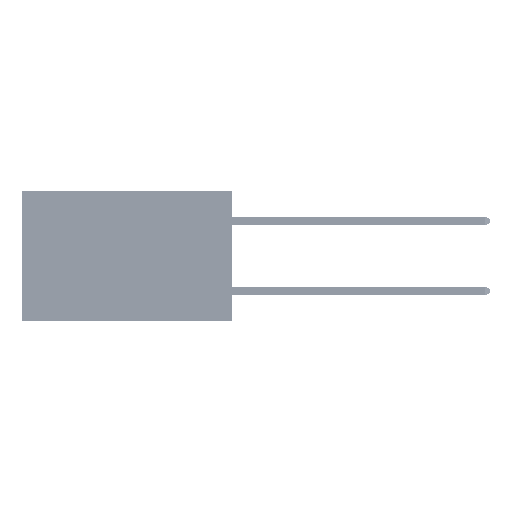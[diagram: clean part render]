
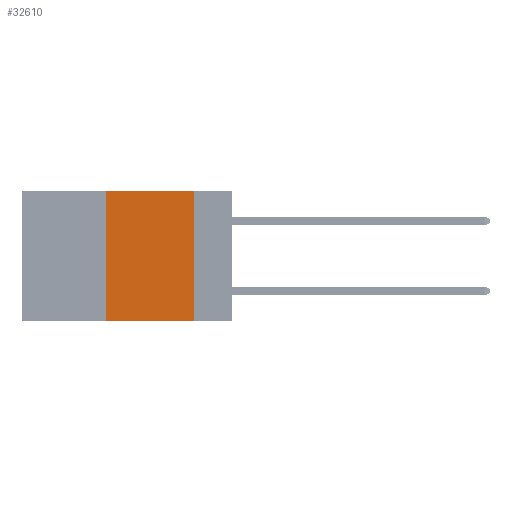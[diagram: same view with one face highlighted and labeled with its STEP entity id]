
A CAD part, left-side view. The second image highlights one B-rep face of the part: STEP entity #32610.
In plain terms, the highlighted planar face has unit normal (-1, 0, 0).
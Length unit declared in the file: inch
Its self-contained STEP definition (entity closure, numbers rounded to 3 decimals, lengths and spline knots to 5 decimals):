
#303 = VERTEX_POINT ( 'NONE', #32655 ) ;
#899 = VERTEX_POINT ( 'NONE', #17360 ) ;
#1774 = EDGE_CURVE ( 'NONE', #899, #2151, #41658, .T. ) ;
#2151 = VERTEX_POINT ( 'NONE', #49190 ) ;
#3017 = CARTESIAN_POINT ( 'NONE',  ( 0., 0.11, 0. ) ) ;
#7585 = DIRECTION ( 'NONE',  ( 0., 0., -1. ) ) ;
#8407 = CARTESIAN_POINT ( 'NONE',  ( 0., 0.11, 0. ) ) ;
#9685 = DIRECTION ( 'NONE',  ( 0., 0., -1. ) ) ;
#9857 = CARTESIAN_POINT ( 'NONE',  ( 0., 0.6, 0. ) ) ;
#10698 = DIRECTION ( 'NONE',  ( 0., -1., 0. ) ) ;
#11963 = CARTESIAN_POINT ( 'NONE',  ( 0., 0.6, -0.37 ) ) ;
#12437 = PLANE ( 'NONE',  #39716 ) ;
#16655 = EDGE_CURVE ( 'NONE', #303, #26631, #48270, .T. ) ;
#17286 = ORIENTED_EDGE ( 'NONE', *, *, #16655, .F. ) ;
#17360 = CARTESIAN_POINT ( 'NONE',  ( 0., 0.36, -0.37 ) ) ;
#18866 = ORIENTED_EDGE ( 'NONE', *, *, #30285, .F. ) ;
#19643 = CARTESIAN_POINT ( 'NONE',  ( 0., 0.36, 0. ) ) ;
#21203 = VECTOR ( 'NONE', #31823, 39.37008 ) ;
#21546 = LINE ( 'NONE', #19643, #25155 ) ;
#25155 = VECTOR ( 'NONE', #31364, 39.37008 ) ;
#25934 = ORIENTED_EDGE ( 'NONE', *, *, #48371, .F. ) ;
#26631 = VERTEX_POINT ( 'NONE', #8407 ) ;
#28339 = ORIENTED_EDGE ( 'NONE', *, *, #1774, .T. ) ;
#30285 = EDGE_CURVE ( 'NONE', #899, #303, #21546, .T. ) ;
#31364 = DIRECTION ( 'NONE',  ( 0., 0., 1. ) ) ;
#31823 = DIRECTION ( 'NONE',  ( 0., -1., 0. ) ) ;
#32610 = ADVANCED_FACE ( 'NONE', ( #33301 ), #12437, .F. ) ;
#32655 = CARTESIAN_POINT ( 'NONE',  ( 0., 0.36, 0. ) ) ;
#33301 = FACE_OUTER_BOUND ( 'NONE', #46955, .T. ) ;
#33748 = CARTESIAN_POINT ( 'NONE',  ( 0., 0.6, 0. ) ) ;
#37980 = VECTOR ( 'NONE', #10698, 39.37008 ) ;
#39716 = AXIS2_PLACEMENT_3D ( 'NONE', #9857, #48492, #9685 ) ;
#40069 = VECTOR ( 'NONE', #7585, 39.37008 ) ;
#41658 = LINE ( 'NONE', #11963, #21203 ) ;
#46955 = EDGE_LOOP ( 'NONE', ( #25934, #17286, #18866, #28339 ) ) ;
#48270 = LINE ( 'NONE', #33748, #37980 ) ;
#48371 = EDGE_CURVE ( 'NONE', #26631, #2151, #49111, .T. ) ;
#48492 = DIRECTION ( 'NONE',  ( 1., 0., 0. ) ) ;
#49111 = LINE ( 'NONE', #3017, #40069 ) ;
#49190 = CARTESIAN_POINT ( 'NONE',  ( 0., 0.11, -0.37 ) ) ;
